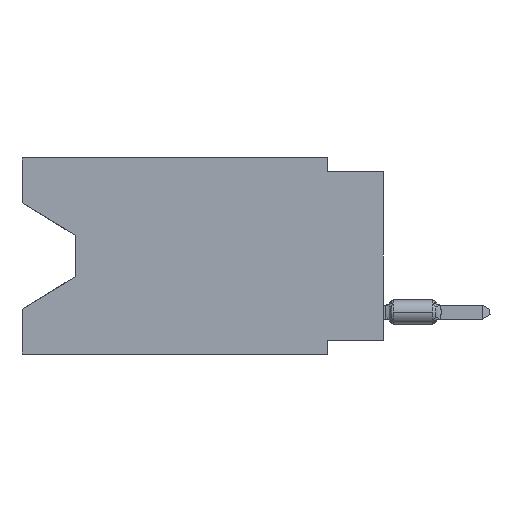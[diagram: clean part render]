
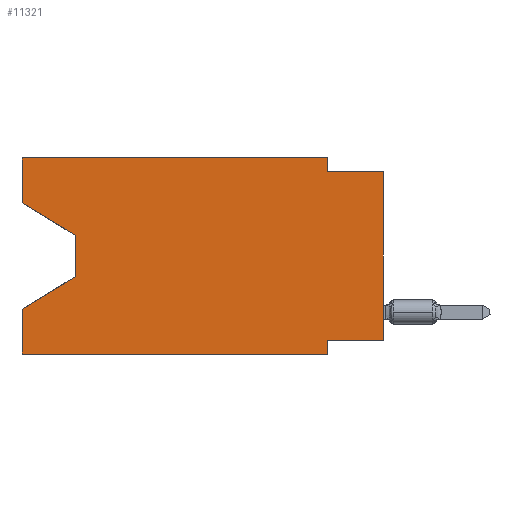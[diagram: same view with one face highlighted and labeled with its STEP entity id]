
A CAD part, left-side view. The second image highlights one B-rep face of the part: STEP entity #11321.
In plain terms, the highlighted planar face has unit normal (-1, 0, 0).
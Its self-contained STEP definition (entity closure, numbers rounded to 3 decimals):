
#208 = CARTESIAN_POINT ( 'NONE',  ( 0., 0., 0. ) ) ;
#1272 = ORIENTED_EDGE ( 'NONE', *, *, #73584, .F. ) ;
#1992 = VERTEX_POINT ( 'NONE', #93724 ) ;
#2250 = LINE ( 'NONE', #38594, #30196 ) ;
#2574 = VECTOR ( 'NONE', #58322, 1000. ) ;
#5606 = CARTESIAN_POINT ( 'NONE',  ( 0., 2.54, -8.89 ) ) ;
#6378 = CARTESIAN_POINT ( 'NONE',  ( 0., 16.383, -6.852 ) ) ;
#7136 = CARTESIAN_POINT ( 'NONE',  ( 0., 0., -0.635 ) ) ;
#7513 = CARTESIAN_POINT ( 'NONE',  ( 0., 13.97, -3.505 ) ) ;
#8420 = CARTESIAN_POINT ( 'NONE',  ( 0., 16.383, 0. ) ) ;
#8495 = CARTESIAN_POINT ( 'NONE',  ( 0., 13.97, -5.385 ) ) ;
#9975 = LINE ( 'NONE', #55242, #45480 ) ;
#10197 = CARTESIAN_POINT ( 'NONE',  ( 0., 16.383, 0. ) ) ;
#10415 = EDGE_LOOP ( 'NONE', ( #52999, #40394, #110606, #1272, #84076, #33100, #79685, #15257, #31454, #93308, #41856, #21911 ) ) ;
#11163 = EDGE_CURVE ( 'NONE', #65042, #102272, #9975, .T. ) ;
#11321 = ADVANCED_FACE ( 'NONE', ( #101694 ), #20064, .F. ) ;
#14874 = EDGE_CURVE ( 'NONE', #84972, #106127, #32165, .T. ) ;
#15257 = ORIENTED_EDGE ( 'NONE', *, *, #110959, .T. ) ;
#17500 = DIRECTION ( 'NONE',  ( 0., 0., 1. ) ) ;
#17892 = DIRECTION ( 'NONE',  ( 0., -0.855, -0.519 ) ) ;
#20064 = PLANE ( 'NONE',  #70152 ) ;
#20868 = DIRECTION ( 'NONE',  ( 0., 0., 1. ) ) ;
#21911 = ORIENTED_EDGE ( 'NONE', *, *, #39334, .F. ) ;
#22553 = CARTESIAN_POINT ( 'NONE',  ( 0., 0., -8.255 ) ) ;
#22757 = LINE ( 'NONE', #97675, #25503 ) ;
#25503 = VECTOR ( 'NONE', #80385, 1000. ) ;
#28110 = VERTEX_POINT ( 'NONE', #49031 ) ;
#30196 = VECTOR ( 'NONE', #92228, 1000. ) ;
#31454 = ORIENTED_EDGE ( 'NONE', *, *, #73590, .F. ) ;
#31871 = DIRECTION ( 'NONE',  ( 0., 0., -1. ) ) ;
#32165 = LINE ( 'NONE', #77437, #96755 ) ;
#33100 = ORIENTED_EDGE ( 'NONE', *, *, #61149, .F. ) ;
#33357 = DIRECTION ( 'NONE',  ( 0., 0.855, -0.519 ) ) ;
#34898 = VERTEX_POINT ( 'NONE', #45220 ) ;
#35303 = VERTEX_POINT ( 'NONE', #37884 ) ;
#37884 = CARTESIAN_POINT ( 'NONE',  ( 0., 2.54, -0.635 ) ) ;
#38594 = CARTESIAN_POINT ( 'NONE',  ( 0., 16.383, 0. ) ) ;
#39334 = EDGE_CURVE ( 'NONE', #93918, #95239, #110287, .T. ) ;
#40231 = CARTESIAN_POINT ( 'NONE',  ( 0., 2.54, 0. ) ) ;
#40394 = ORIENTED_EDGE ( 'NONE', *, *, #74319, .T. ) ;
#41035 = LINE ( 'NONE', #48797, #2574 ) ;
#41856 = ORIENTED_EDGE ( 'NONE', *, *, #60093, .F. ) ;
#41951 = DIRECTION ( 'NONE',  ( 0., 0., -1. ) ) ;
#42552 = VECTOR ( 'NONE', #83994, 1000. ) ;
#43859 = LINE ( 'NONE', #7513, #84475 ) ;
#44709 = LINE ( 'NONE', #117393, #83988 ) ;
#45220 = CARTESIAN_POINT ( 'NONE',  ( 0., 13.97, -3.505 ) ) ;
#45480 = VECTOR ( 'NONE', #109474, 1000. ) ;
#48797 = CARTESIAN_POINT ( 'NONE',  ( 0., 16.383, 0. ) ) ;
#49031 = CARTESIAN_POINT ( 'NONE',  ( 0., 2.54, 0. ) ) ;
#50202 = CARTESIAN_POINT ( 'NONE',  ( 0., 2.54, -8.89 ) ) ;
#50475 = CARTESIAN_POINT ( 'NONE',  ( 0., 2.54, -8.255 ) ) ;
#52999 = ORIENTED_EDGE ( 'NONE', *, *, #69365, .T. ) ;
#55242 = CARTESIAN_POINT ( 'NONE',  ( 0., 0., -8.255 ) ) ;
#56392 = DIRECTION ( 'NONE',  ( 1., 0., 0. ) ) ;
#58322 = DIRECTION ( 'NONE',  ( 0., 0., 1. ) ) ;
#60093 = EDGE_CURVE ( 'NONE', #95239, #28110, #2250, .T. ) ;
#61149 = EDGE_CURVE ( 'NONE', #102272, #113589, #87233, .T. ) ;
#65042 = VERTEX_POINT ( 'NONE', #22553 ) ;
#65917 = CARTESIAN_POINT ( 'NONE',  ( 0., 16.383, 0. ) ) ;
#69365 = EDGE_CURVE ( 'NONE', #93918, #34898, #44709, .T. ) ;
#70152 = AXIS2_PLACEMENT_3D ( 'NONE', #65917, #56392, #74883 ) ;
#73584 = EDGE_CURVE ( 'NONE', #1992, #106127, #41035, .T. ) ;
#73590 = EDGE_CURVE ( 'NONE', #35303, #108865, #85154, .T. ) ;
#74319 = EDGE_CURVE ( 'NONE', #34898, #84972, #43859, .T. ) ;
#74883 = DIRECTION ( 'NONE',  ( 0., 0., -1. ) ) ;
#77437 = CARTESIAN_POINT ( 'NONE',  ( 0., 13.97, -5.385 ) ) ;
#79685 = ORIENTED_EDGE ( 'NONE', *, *, #11163, .F. ) ;
#80385 = DIRECTION ( 'NONE',  ( 0., -1., 0. ) ) ;
#81905 = EDGE_CURVE ( 'NONE', #28110, #35303, #84353, .T. ) ;
#83988 = VECTOR ( 'NONE', #17892, 1000. ) ;
#83994 = DIRECTION ( 'NONE',  ( 0., -1., 0. ) ) ;
#84076 = ORIENTED_EDGE ( 'NONE', *, *, #111295, .T. ) ;
#84353 = LINE ( 'NONE', #40231, #90780 ) ;
#84475 = VECTOR ( 'NONE', #89737, 1000. ) ;
#84972 = VERTEX_POINT ( 'NONE', #8495 ) ;
#85154 = LINE ( 'NONE', #94088, #42552 ) ;
#87233 = LINE ( 'NONE', #5606, #91211 ) ;
#89737 = DIRECTION ( 'NONE',  ( 0., 0., -1. ) ) ;
#90780 = VECTOR ( 'NONE', #31871, 1000. ) ;
#91211 = VECTOR ( 'NONE', #41951, 1000. ) ;
#91364 = LINE ( 'NONE', #208, #111060 ) ;
#91413 = CARTESIAN_POINT ( 'NONE',  ( 0., 16.383, -2.038 ) ) ;
#92228 = DIRECTION ( 'NONE',  ( 0., -1., 0. ) ) ;
#93308 = ORIENTED_EDGE ( 'NONE', *, *, #81905, .F. ) ;
#93724 = CARTESIAN_POINT ( 'NONE',  ( 0., 16.383, -8.89 ) ) ;
#93918 = VERTEX_POINT ( 'NONE', #91413 ) ;
#94088 = CARTESIAN_POINT ( 'NONE',  ( 0., 0., -0.635 ) ) ;
#95239 = VERTEX_POINT ( 'NONE', #8420 ) ;
#96755 = VECTOR ( 'NONE', #33357, 1000. ) ;
#97675 = CARTESIAN_POINT ( 'NONE',  ( 0., 16.383, -8.89 ) ) ;
#98214 = VECTOR ( 'NONE', #20868, 1000. ) ;
#101694 = FACE_OUTER_BOUND ( 'NONE', #10415, .T. ) ;
#102272 = VERTEX_POINT ( 'NONE', #50475 ) ;
#106127 = VERTEX_POINT ( 'NONE', #6378 ) ;
#108865 = VERTEX_POINT ( 'NONE', #7136 ) ;
#109474 = DIRECTION ( 'NONE',  ( 0., 1., 0. ) ) ;
#110287 = LINE ( 'NONE', #10197, #98214 ) ;
#110606 = ORIENTED_EDGE ( 'NONE', *, *, #14874, .T. ) ;
#110959 = EDGE_CURVE ( 'NONE', #65042, #108865, #91364, .T. ) ;
#111060 = VECTOR ( 'NONE', #17500, 1000. ) ;
#111295 = EDGE_CURVE ( 'NONE', #1992, #113589, #22757, .T. ) ;
#113589 = VERTEX_POINT ( 'NONE', #50202 ) ;
#117393 = CARTESIAN_POINT ( 'NONE',  ( 0., 16.383, -2.038 ) ) ;
